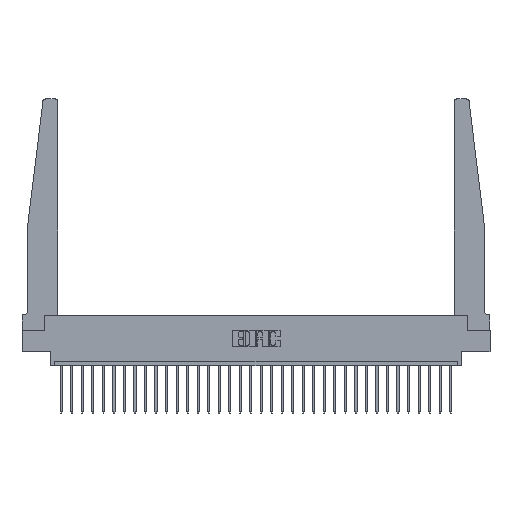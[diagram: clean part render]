
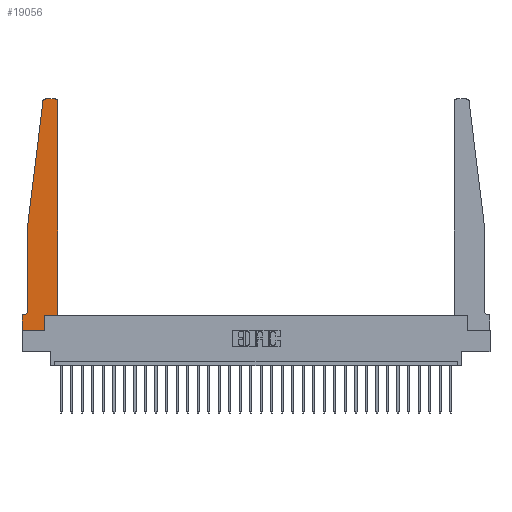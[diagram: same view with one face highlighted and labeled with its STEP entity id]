
A CAD part, top view. The second image highlights one B-rep face of the part: STEP entity #19056.
In plain terms, the highlighted planar face has unit normal (0, 0, 1).
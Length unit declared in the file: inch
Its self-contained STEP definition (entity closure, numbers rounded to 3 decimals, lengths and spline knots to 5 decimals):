
#131 = VECTOR ( 'NONE', #16563, 39.37008 ) ;
#895 = VECTOR ( 'NONE', #17345, 39.37008 ) ;
#1766 = CIRCLE ( 'NONE', #18417, 0.05 ) ;
#2021 = VERTEX_POINT ( 'NONE', #8452 ) ;
#2857 = CARTESIAN_POINT ( 'NONE',  ( 0.015, 0.2375, 0.37 ) ) ;
#3480 = EDGE_CURVE ( 'NONE', #8913, #11333, #17790, .T. ) ;
#3779 = DIRECTION ( 'NONE',  ( -1., 0., 0. ) ) ;
#4999 = EDGE_CURVE ( 'NONE', #9214, #18829, #19413, .T. ) ;
#5090 = ORIENTED_EDGE ( 'NONE', *, *, #19587, .T. ) ;
#5235 = CIRCLE ( 'NONE', #11873, 0.03 ) ;
#5268 = CARTESIAN_POINT ( 'NONE',  ( 0.065, 1.25, 0.37 ) ) ;
#5342 = CIRCLE ( 'NONE', #19607, 0.03 ) ;
#5447 = LINE ( 'NONE', #14489, #5712 ) ;
#5453 = CARTESIAN_POINT ( 'NONE',  ( 0.425, 0.18, 0.37 ) ) ;
#5541 = VECTOR ( 'NONE', #3779, 39.37008 ) ;
#5694 = ORIENTED_EDGE ( 'NONE', *, *, #10527, .T. ) ;
#5712 = VECTOR ( 'NONE', #25417, 39.37008 ) ;
#5736 = CARTESIAN_POINT ( 'NONE',  ( 0.27653, 2.72, 0.37 ) ) ;
#5768 = CARTESIAN_POINT ( 'NONE',  ( 0.065, 1.25, 0.37 ) ) ;
#6947 = DIRECTION ( 'NONE',  ( 0., 0., 1. ) ) ;
#7173 = ORIENTED_EDGE ( 'NONE', *, *, #18854, .T. ) ;
#7704 = DIRECTION ( 'NONE',  ( 1., 0., 0. ) ) ;
#8023 = ORIENTED_EDGE ( 'NONE', *, *, #4999, .T. ) ;
#8037 = ORIENTED_EDGE ( 'NONE', *, *, #24149, .T. ) ;
#8258 = EDGE_CURVE ( 'NONE', #19971, #2021, #1766, .T. ) ;
#8452 = CARTESIAN_POINT ( 'NONE',  ( 0.015, 0.1875, 0.37 ) ) ;
#8913 = VERTEX_POINT ( 'NONE', #22628 ) ;
#9002 = VECTOR ( 'NONE', #27193, 39.37008 ) ;
#9214 = VERTEX_POINT ( 'NONE', #10240 ) ;
#9322 = DIRECTION ( 'NONE',  ( -0.122, -0.992, 0. ) ) ;
#9520 = PLANE ( 'NONE',  #21874 ) ;
#9817 = VECTOR ( 'NONE', #20780, 39.37008 ) ;
#9881 = VERTEX_POINT ( 'NONE', #10500 ) ;
#10195 = DIRECTION ( 'NONE',  ( 0., 0., 1. ) ) ;
#10240 = CARTESIAN_POINT ( 'NONE',  ( 0.395, 2.75, 0.37 ) ) ;
#10500 = CARTESIAN_POINT ( 'NONE',  ( 0.2605, 0., 0.37 ) ) ;
#10527 = EDGE_CURVE ( 'NONE', #24917, #9881, #11891, .T. ) ;
#10986 = EDGE_CURVE ( 'NONE', #22443, #24917, #5447, .T. ) ;
#11333 = VERTEX_POINT ( 'NONE', #5268 ) ;
#11873 = AXIS2_PLACEMENT_3D ( 'NONE', #5736, #10195, #28370 ) ;
#11891 = LINE ( 'NONE', #20986, #18033 ) ;
#12176 = DIRECTION ( 'NONE',  ( 1., 0., 0. ) ) ;
#12314 = VERTEX_POINT ( 'NONE', #5453 ) ;
#12712 = CARTESIAN_POINT ( 'NONE',  ( 0.27653, 2.75, 0.37 ) ) ;
#13901 = LINE ( 'NONE', #18804, #131 ) ;
#14029 = DIRECTION ( 'NONE',  ( -1., 0., 0. ) ) ;
#14098 = VERTEX_POINT ( 'NONE', #26695 ) ;
#14224 = VERTEX_POINT ( 'NONE', #22984 ) ;
#14489 = CARTESIAN_POINT ( 'NONE',  ( 0., 0., 0.37 ) ) ;
#14531 = ORIENTED_EDGE ( 'NONE', *, *, #18628, .T. ) ;
#15003 = EDGE_LOOP ( 'NONE', ( #8023, #7173, #22191, #18881, #17410, #14531, #27997, #5694, #8037, #5090, #27088, #15056 ) ) ;
#15056 = ORIENTED_EDGE ( 'NONE', *, *, #15754, .T. ) ;
#15754 = EDGE_CURVE ( 'NONE', #14098, #9214, #5342, .T. ) ;
#15986 = DIRECTION ( 'NONE',  ( 1., 0., 0. ) ) ;
#15999 = LINE ( 'NONE', #25118, #9817 ) ;
#16563 = DIRECTION ( 'NONE',  ( 0., 1., 0. ) ) ;
#16630 = FACE_OUTER_BOUND ( 'NONE', #15003, .T. ) ;
#16891 = CARTESIAN_POINT ( 'NONE',  ( 0., 0., 0.37 ) ) ;
#17345 = DIRECTION ( 'NONE',  ( 0., -1., 0. ) ) ;
#17410 = ORIENTED_EDGE ( 'NONE', *, *, #8258, .T. ) ;
#17790 = LINE ( 'NONE', #20326, #18293 ) ;
#18033 = VECTOR ( 'NONE', #27842, 39.37008 ) ;
#18293 = VECTOR ( 'NONE', #9322, 39.37008 ) ;
#18417 = AXIS2_PLACEMENT_3D ( 'NONE', #2857, #21050, #14029 ) ;
#18510 = EDGE_CURVE ( 'NONE', #11333, #19971, #26458, .T. ) ;
#18628 = EDGE_CURVE ( 'NONE', #2021, #22443, #20178, .T. ) ;
#18700 = LINE ( 'NONE', #23336, #28560 ) ;
#18804 = CARTESIAN_POINT ( 'NONE',  ( 0.2605, 0.18, 0.37 ) ) ;
#18829 = VERTEX_POINT ( 'NONE', #12712 ) ;
#18854 = EDGE_CURVE ( 'NONE', #18829, #8913, #5235, .T. ) ;
#18881 = ORIENTED_EDGE ( 'NONE', *, *, #18510, .T. ) ;
#19056 = ADVANCED_FACE ( 'NONE', ( #16630 ), #9520, .T. ) ;
#19413 = LINE ( 'NONE', #26130, #5541 ) ;
#19587 = EDGE_CURVE ( 'NONE', #14224, #12314, #18700, .T. ) ;
#19607 = AXIS2_PLACEMENT_3D ( 'NONE', #24401, #6947, #15986 ) ;
#19971 = VERTEX_POINT ( 'NONE', #21206 ) ;
#20178 = LINE ( 'NONE', #24656, #9002 ) ;
#20326 = CARTESIAN_POINT ( 'NONE',  ( 0.065, 1.25, 0.37 ) ) ;
#20780 = DIRECTION ( 'NONE',  ( 0., 1., 0. ) ) ;
#20986 = CARTESIAN_POINT ( 'NONE',  ( 0., 0., 0.37 ) ) ;
#21050 = DIRECTION ( 'NONE',  ( 0., 0., -1. ) ) ;
#21130 = CARTESIAN_POINT ( 'NONE',  ( 0., 0.1875, 0.37 ) ) ;
#21206 = CARTESIAN_POINT ( 'NONE',  ( 0.065, 0.2375, 0.37 ) ) ;
#21419 = DIRECTION ( 'NONE',  ( 0., 0., 1. ) ) ;
#21874 = AXIS2_PLACEMENT_3D ( 'NONE', #21130, #21419, #12176 ) ;
#22191 = ORIENTED_EDGE ( 'NONE', *, *, #3480, .T. ) ;
#22443 = VERTEX_POINT ( 'NONE', #27224 ) ;
#22628 = CARTESIAN_POINT ( 'NONE',  ( 0.24675, 2.72367, 0.37 ) ) ;
#22984 = CARTESIAN_POINT ( 'NONE',  ( 0.2605, 0.18, 0.37 ) ) ;
#23336 = CARTESIAN_POINT ( 'NONE',  ( 0.425, 0.18, 0.37 ) ) ;
#24149 = EDGE_CURVE ( 'NONE', #9881, #14224, #13901, .T. ) ;
#24401 = CARTESIAN_POINT ( 'NONE',  ( 0.395, 2.72, 0.37 ) ) ;
#24656 = CARTESIAN_POINT ( 'NONE',  ( 0.065, 0.1875, 0.37 ) ) ;
#24917 = VERTEX_POINT ( 'NONE', #16891 ) ;
#25118 = CARTESIAN_POINT ( 'NONE',  ( 0.425, 0.18, 0.37 ) ) ;
#25417 = DIRECTION ( 'NONE',  ( 0., -1., 0. ) ) ;
#26130 = CARTESIAN_POINT ( 'NONE',  ( 0.25, 2.75, 0.37 ) ) ;
#26458 = LINE ( 'NONE', #5768, #895 ) ;
#26695 = CARTESIAN_POINT ( 'NONE',  ( 0.425, 2.72, 0.37 ) ) ;
#27088 = ORIENTED_EDGE ( 'NONE', *, *, #28326, .T. ) ;
#27193 = DIRECTION ( 'NONE',  ( -1., 0., 0. ) ) ;
#27224 = CARTESIAN_POINT ( 'NONE',  ( 0., 0.1875, 0.37 ) ) ;
#27842 = DIRECTION ( 'NONE',  ( 1., 0., 0. ) ) ;
#27997 = ORIENTED_EDGE ( 'NONE', *, *, #10986, .T. ) ;
#28326 = EDGE_CURVE ( 'NONE', #12314, #14098, #15999, .T. ) ;
#28370 = DIRECTION ( 'NONE',  ( 1., 0., 0. ) ) ;
#28560 = VECTOR ( 'NONE', #7704, 39.37008 ) ;
